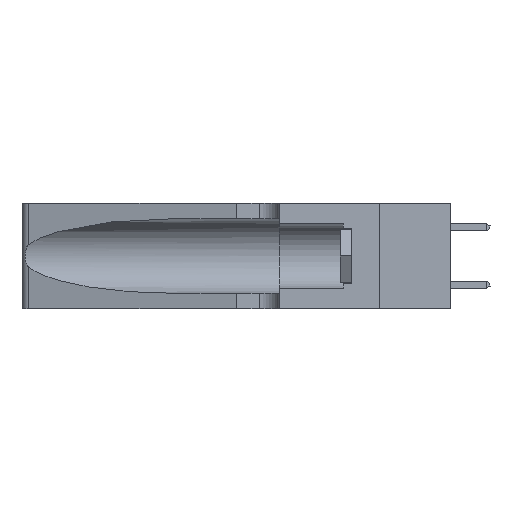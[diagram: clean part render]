
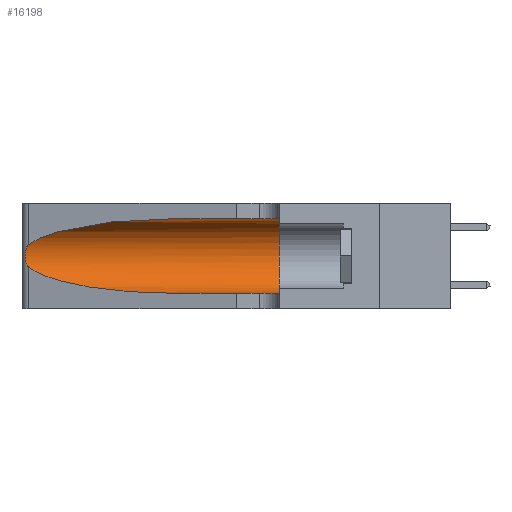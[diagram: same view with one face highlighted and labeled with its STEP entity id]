
A CAD part, left-side view. The second image highlights one B-rep face of the part: STEP entity #16198.
In plain terms, the highlighted cylindrical face has radius 3.308 mm (diameter 6.617 mm), a partial arc.
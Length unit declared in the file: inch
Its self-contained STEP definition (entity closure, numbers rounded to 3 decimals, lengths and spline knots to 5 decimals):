
#807 = CARTESIAN_POINT ( 'NONE',  ( 0.1305, 0.35, 0.05475 ) ) ;
#1308 = CARTESIAN_POINT ( 'NONE',  ( 0.25555, 1.22994, 0.2215 ) ) ;
#1368 = CARTESIAN_POINT ( 'NONE',  ( 0.25487, 1.22718, 0.14631 ) ) ;
#2129 = VERTEX_POINT ( 'NONE', #14127 ) ;
#2493 = DIRECTION ( 'NONE',  ( 0., -1., 0. ) ) ;
#2673 = CARTESIAN_POINT ( 'NONE',  ( 0.25639, 1.23184, 0.21858 ) ) ;
#3532 = CARTESIAN_POINT ( 'NONE',  ( 0.1305, 1.61858, 0.05475 ) ) ;
#3621 = CARTESIAN_POINT ( 'NONE',  ( 0.25487, 1.22718, 0.22369 ) ) ;
#3876 = LINE ( 'NONE', #3532, #6638 ) ;
#4045 = CARTESIAN_POINT ( 'NONE',  ( 0.25854, 1.2359, 0.20912 ) ) ;
#4073 = EDGE_CURVE ( 'NONE', #13321, #5987, #12049, .T. ) ;
#4202 = EDGE_CURVE ( 'NONE', #5987, #11990, #3876, .T. ) ;
#4418 = DIRECTION ( 'NONE',  ( 0., -1., 0. ) ) ;
#4610 = CARTESIAN_POINT ( 'NONE',  ( 0.18966, 0.96281, 0.05475 ) ) ;
#4773 = ORIENTED_EDGE ( 'NONE', *, *, #11586, .T. ) ;
#4879 = ORIENTED_EDGE ( 'NONE', *, *, #8921, .F. ) ;
#5420 = CARTESIAN_POINT ( 'NONE',  ( 0.26075, 1.23896, 0.19203 ) ) ;
#5874 = VERTEX_POINT ( 'NONE', #8934 ) ;
#5987 = VERTEX_POINT ( 'NONE', #10607 ) ;
#5995 = CYLINDRICAL_SURFACE ( 'NONE', #7538, 0.13025 ) ;
#6423 = FACE_OUTER_BOUND ( 'NONE', #12607, .T. ) ;
#6449 = ORIENTED_EDGE ( 'NONE', *, *, #4202, .T. ) ;
#6542 = DIRECTION ( 'NONE',  ( 0., 1., 0. ) ) ;
#6638 = VECTOR ( 'NONE', #14410, 39.37008 ) ;
#6778 = CARTESIAN_POINT ( 'NONE',  ( 0.26017, 1.23833, 0.17102 ) ) ;
#6877 = VERTEX_POINT ( 'NONE', #8715 ) ;
#7337 = CARTESIAN_POINT ( 'NONE',  ( 0.25487, 1.22718, 0.14631 ) ) ;
#7538 = AXIS2_PLACEMENT_3D ( 'NONE', #8440, #4418, #13932 ) ;
#7656 = CARTESIAN_POINT ( 'NONE',  ( 0.18966, 0.96281, 0.31525 ) ) ;
#8141 = CARTESIAN_POINT ( 'NONE',  ( 0.25789, 1.23486, 0.15765 ) ) ;
#8440 = CARTESIAN_POINT ( 'NONE',  ( 0.1305, 1.61858, 0.185 ) ) ;
#8715 = CARTESIAN_POINT ( 'NONE',  ( 0.25487, 1.22718, 0.22369 ) ) ;
#8917 = LINE ( 'NONE', #10634, #11700 ) ;
#8921 = EDGE_CURVE ( 'NONE', #2129, #11990, #16904, .T. ) ;
#8934 = CARTESIAN_POINT ( 'NONE',  ( 0.1305, 0.72297, 0.31525 ) ) ;
#9505 = CARTESIAN_POINT ( 'NONE',  ( 0.25555, 1.22993, 0.14849 ) ) ;
#10086 =( BOUNDED_CURVE ( )  B_SPLINE_CURVE ( 3, ( #17153, #7656, #11774, #3621 ),
 .UNSPECIFIED., .F., .F. ) 
 B_SPLINE_CURVE_WITH_KNOTS ( ( 4, 4 ),
 ( 1.5708, 2.84003 ),
 .UNSPECIFIED. ) 
 CURVE ( )  GEOMETRIC_REPRESENTATION_ITEM ( )  RATIONAL_B_SPLINE_CURVE ( ( 1., 0.87, 0.87, 1. ) ) 
 REPRESENTATION_ITEM ( '' )  );
#10607 = CARTESIAN_POINT ( 'NONE',  ( 0.1305, 0.72297, 0.05475 ) ) ;
#10634 = CARTESIAN_POINT ( 'NONE',  ( 0.1305, 1.61858, 0.31525 ) ) ;
#10819 = CARTESIAN_POINT ( 'NONE',  ( 0.25487, 1.22718, 0.22369 ) ) ;
#10828 = ORIENTED_EDGE ( 'NONE', *, *, #11474, .F. ) ;
#11331 = ORIENTED_EDGE ( 'NONE', *, *, #11352, .T. ) ;
#11352 = EDGE_CURVE ( 'NONE', #5874, #6877, #10086, .T. ) ;
#11445 = AXIS2_PLACEMENT_3D ( 'NONE', #14670, #6542, #16031 ) ;
#11463 = CARTESIAN_POINT ( 'NONE',  ( 0.25639, 1.23186, 0.15144 ) ) ;
#11474 = EDGE_CURVE ( 'NONE', #5874, #2129, #8917, .T. ) ;
#11586 = EDGE_CURVE ( 'NONE', #6877, #13321, #17146, .T. ) ;
#11700 = VECTOR ( 'NONE', #2493, 39.37008 ) ;
#11774 = CARTESIAN_POINT ( 'NONE',  ( 0.2373, 1.15595, 0.28018 ) ) ;
#11990 = VERTEX_POINT ( 'NONE', #807 ) ;
#12049 =( BOUNDED_CURVE ( )  B_SPLINE_CURVE ( 3, ( #7337, #15454, #4610, #16830 ),
 .UNSPECIFIED., .F., .T. ) 
 B_SPLINE_CURVE_WITH_KNOTS ( ( 4, 4 ),
 ( 3.44316, 4.71239 ),
 .UNSPECIFIED. ) 
 CURVE ( )  GEOMETRIC_REPRESENTATION_ITEM ( )  RATIONAL_B_SPLINE_CURVE ( ( 1., 0.87, 0.87, 1. ) ) 
 REPRESENTATION_ITEM ( '' )  );
#12196 = CARTESIAN_POINT ( 'NONE',  ( 0.25787, 1.23484, 0.2124 ) ) ;
#12607 = EDGE_LOOP ( 'NONE', ( #11331, #4773, #15394, #6449, #4879, #10828 ) ) ;
#13321 = VERTEX_POINT ( 'NONE', #13325 ) ;
#13325 = CARTESIAN_POINT ( 'NONE',  ( 0.25487, 1.22718, 0.14631 ) ) ;
#13567 = CARTESIAN_POINT ( 'NONE',  ( 0.26018, 1.23835, 0.19895 ) ) ;
#13932 = DIRECTION ( 'NONE',  ( 0., 0., -1. ) ) ;
#14127 = CARTESIAN_POINT ( 'NONE',  ( 0.1305, 0.35, 0.31525 ) ) ;
#14410 = DIRECTION ( 'NONE',  ( 0., -1., 0. ) ) ;
#14670 = CARTESIAN_POINT ( 'NONE',  ( 0.1305, 0.35, 0.185 ) ) ;
#14907 = CARTESIAN_POINT ( 'NONE',  ( 0.26075, 1.23896, 0.178 ) ) ;
#15394 = ORIENTED_EDGE ( 'NONE', *, *, #4073, .T. ) ;
#15454 = CARTESIAN_POINT ( 'NONE',  ( 0.2373, 1.15595, 0.08982 ) ) ;
#16031 = DIRECTION ( 'NONE',  ( 0., 0., 1. ) ) ;
#16198 = ADVANCED_FACE ( 'NONE', ( #6423 ), #5995, .F. ) ;
#16274 = CARTESIAN_POINT ( 'NONE',  ( 0.25856, 1.23593, 0.16098 ) ) ;
#16830 = CARTESIAN_POINT ( 'NONE',  ( 0.1305, 0.72297, 0.05475 ) ) ;
#16904 = CIRCLE ( 'NONE', #11445, 0.13025 ) ;
#17146 = B_SPLINE_CURVE_WITH_KNOTS ( 'NONE', 3,
 ( #10819, #1308, #2673, #12196, #4045, #13567, #5420, #14907, #6778, #16274, #8141, #11463, #9505, #1368 ),
 .UNSPECIFIED., .F., .F.,
 ( 4, 2, 2, 2, 2, 2, 4 ),
 ( 0., 0.00027, 0.00053, 0.00107, 0.0016, 0.00187, 0.00214 ),
 .UNSPECIFIED. ) ;
#17153 = CARTESIAN_POINT ( 'NONE',  ( 0.1305, 0.72297, 0.31525 ) ) ;
